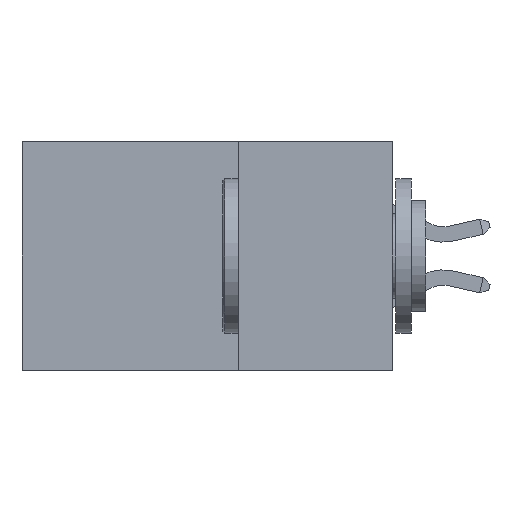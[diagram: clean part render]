
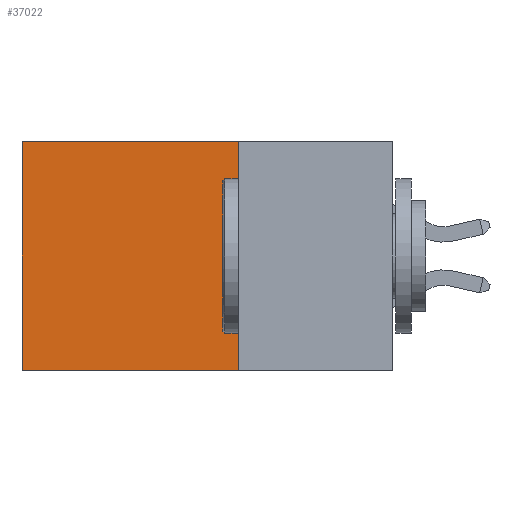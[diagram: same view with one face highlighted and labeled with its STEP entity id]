
A CAD part, left-side view. The second image highlights one B-rep face of the part: STEP entity #37022.
In plain terms, the highlighted planar face has unit normal (-1, 0, 0).
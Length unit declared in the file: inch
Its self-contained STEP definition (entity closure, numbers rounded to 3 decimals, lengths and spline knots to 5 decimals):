
#299 = CARTESIAN_POINT ( 'NONE',  ( 0.2875, 0.6, 0. ) ) ;
#745 = DIRECTION ( 'NONE',  ( 0., 1., 0. ) ) ;
#800 = ORIENTED_EDGE ( 'NONE', *, *, #26190, .F. ) ;
#1515 = EDGE_CURVE ( 'NONE', #24505, #30991, #1746, .T. ) ;
#1746 = LINE ( 'NONE', #33098, #3666 ) ;
#3666 = VECTOR ( 'NONE', #5795, 39.37008 ) ;
#4212 = CARTESIAN_POINT ( 'NONE',  ( 0.2875, 0.25, 0. ) ) ;
#4811 = FACE_OUTER_BOUND ( 'NONE', #13009, .T. ) ;
#5795 = DIRECTION ( 'NONE',  ( 0., 0., -1. ) ) ;
#6057 = EDGE_CURVE ( 'NONE', #24505, #15161, #18363, .T. ) ;
#6324 = VERTEX_POINT ( 'NONE', #38895 ) ;
#7405 = ORIENTED_EDGE ( 'NONE', *, *, #36515, .T. ) ;
#7877 = AXIS2_PLACEMENT_3D ( 'NONE', #26606, #29682, #35021 ) ;
#8844 = VECTOR ( 'NONE', #745, 39.37008 ) ;
#8860 = DIRECTION ( 'NONE',  ( 0., 0., -1. ) ) ;
#8888 = VECTOR ( 'NONE', #15064, 39.37008 ) ;
#11797 = CARTESIAN_POINT ( 'NONE',  ( 0.2875, 0.6, 0. ) ) ;
#13009 = EDGE_LOOP ( 'NONE', ( #7405, #800, #21747, #39604 ) ) ;
#13641 = PLANE ( 'NONE',  #7877 ) ;
#15064 = DIRECTION ( 'NONE',  ( 0., 1., 0. ) ) ;
#15161 = VERTEX_POINT ( 'NONE', #299 ) ;
#16820 = LINE ( 'NONE', #11797, #38885 ) ;
#16985 = LINE ( 'NONE', #39011, #8888 ) ;
#18363 = LINE ( 'NONE', #34221, #8844 ) ;
#21747 = ORIENTED_EDGE ( 'NONE', *, *, #1515, .F. ) ;
#24505 = VERTEX_POINT ( 'NONE', #4212 ) ;
#26190 = EDGE_CURVE ( 'NONE', #30991, #6324, #16985, .T. ) ;
#26606 = CARTESIAN_POINT ( 'NONE',  ( 0.2875, 0.25, 0. ) ) ;
#29682 = DIRECTION ( 'NONE',  ( 1., 0., 0. ) ) ;
#30991 = VERTEX_POINT ( 'NONE', #33072 ) ;
#33072 = CARTESIAN_POINT ( 'NONE',  ( 0.2875, 0.25, -0.37 ) ) ;
#33098 = CARTESIAN_POINT ( 'NONE',  ( 0.2875, 0.25, 0. ) ) ;
#34221 = CARTESIAN_POINT ( 'NONE',  ( 0.2875, 0.25, 0. ) ) ;
#35021 = DIRECTION ( 'NONE',  ( 0., 0., -1. ) ) ;
#36515 = EDGE_CURVE ( 'NONE', #15161, #6324, #16820, .T. ) ;
#37022 = ADVANCED_FACE ( 'NONE', ( #4811 ), #13641, .F. ) ;
#38885 = VECTOR ( 'NONE', #8860, 39.37008 ) ;
#38895 = CARTESIAN_POINT ( 'NONE',  ( 0.2875, 0.6, -0.37 ) ) ;
#39011 = CARTESIAN_POINT ( 'NONE',  ( 0.2875, 0.25, -0.37 ) ) ;
#39604 = ORIENTED_EDGE ( 'NONE', *, *, #6057, .T. ) ;
